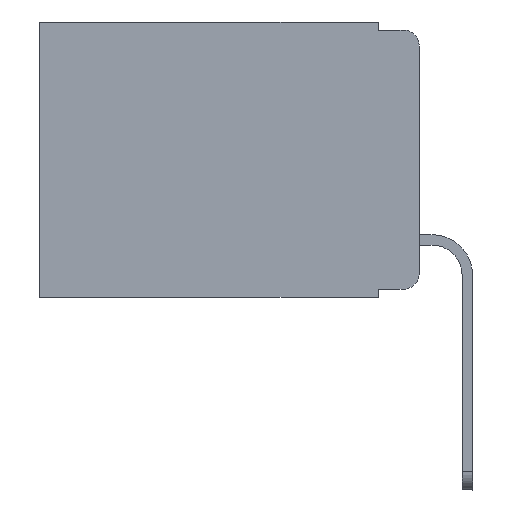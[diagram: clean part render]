
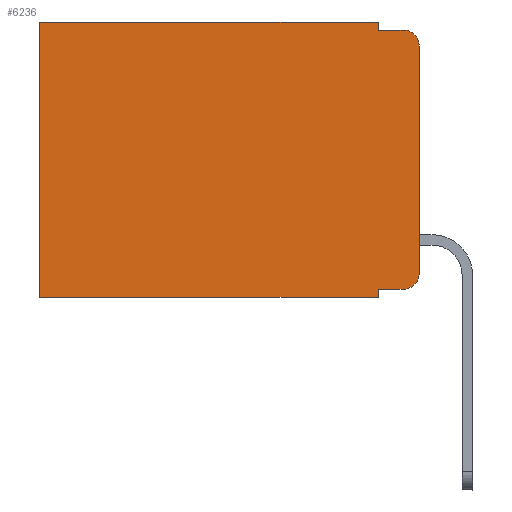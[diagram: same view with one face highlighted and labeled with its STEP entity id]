
A CAD part, left-side view. The second image highlights one B-rep face of the part: STEP entity #6236.
In plain terms, the highlighted planar face has unit normal (-1, 0, 0).
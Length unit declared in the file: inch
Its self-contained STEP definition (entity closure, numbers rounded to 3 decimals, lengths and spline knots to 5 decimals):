
#147 = AXIS2_PLACEMENT_3D ( 'NONE', #1263, #9420, #14792 ) ;
#292 = VECTOR ( 'NONE', #2814, 39.37008 ) ;
#381 = CARTESIAN_POINT ( 'NONE',  ( 0.298, 0., 0. ) ) ;
#407 = CARTESIAN_POINT ( 'NONE',  ( 0.298, 0., -0.03 ) ) ;
#532 = CARTESIAN_POINT ( 'NONE',  ( 0.298, 0.051, -0.333 ) ) ;
#618 = DIRECTION ( 'NONE',  ( 0., 1., 0. ) ) ;
#841 = CARTESIAN_POINT ( 'NONE',  ( 0.298, 0.051, 0. ) ) ;
#1177 = FACE_OUTER_BOUND ( 'NONE', #15107, .T. ) ;
#1263 = CARTESIAN_POINT ( 'NONE',  ( 0.298, 0., 0. ) ) ;
#1312 = DIRECTION ( 'NONE',  ( 0., 0., -1. ) ) ;
#1397 = CARTESIAN_POINT ( 'NONE',  ( 0.298, 0.051, -0.333 ) ) ;
#1492 = CARTESIAN_POINT ( 'NONE',  ( 0.298, 0.051, 0. ) ) ;
#1505 = ORIENTED_EDGE ( 'NONE', *, *, #8779, .F. ) ;
#1575 = VECTOR ( 'NONE', #2455, 39.37008 ) ;
#1596 = CARTESIAN_POINT ( 'NONE',  ( 0.298, 0.02, -0.03 ) ) ;
#1624 = VECTOR ( 'NONE', #5304, 39.37008 ) ;
#1857 = DIRECTION ( 'NONE',  ( 0., -1., 0. ) ) ;
#2455 = DIRECTION ( 'NONE',  ( 0., 0., -1. ) ) ;
#2542 = LINE ( 'NONE', #15718, #1575 ) ;
#2643 = EDGE_CURVE ( 'NONE', #16967, #6027, #7352, .T. ) ;
#2814 = DIRECTION ( 'NONE',  ( 0., 0., -1. ) ) ;
#3098 = ORIENTED_EDGE ( 'NONE', *, *, #8596, .T. ) ;
#3235 = ORIENTED_EDGE ( 'NONE', *, *, #4909, .T. ) ;
#3703 = LINE ( 'NONE', #9099, #292 ) ;
#3715 = EDGE_CURVE ( 'NONE', #4102, #5223, #4600, .T. ) ;
#3789 = CARTESIAN_POINT ( 'NONE',  ( 0.298, 0.02, -0.333 ) ) ;
#3904 = CARTESIAN_POINT ( 'NONE',  ( 0.298, 0., -0.313 ) ) ;
#3988 = EDGE_CURVE ( 'NONE', #6385, #6027, #17222, .T. ) ;
#4102 = VERTEX_POINT ( 'NONE', #1397 ) ;
#4171 = CIRCLE ( 'NONE', #8983, 0.02 ) ;
#4177 = CIRCLE ( 'NONE', #4748, 0.02 ) ;
#4514 = ORIENTED_EDGE ( 'NONE', *, *, #14422, .F. ) ;
#4600 = LINE ( 'NONE', #532, #14358 ) ;
#4748 = AXIS2_PLACEMENT_3D ( 'NONE', #1596, #9482, #13632 ) ;
#4909 = EDGE_CURVE ( 'NONE', #12783, #16648, #4177, .T. ) ;
#4951 = DIRECTION ( 'NONE',  ( -1., 0., 0. ) ) ;
#5069 = CARTESIAN_POINT ( 'NONE',  ( 0.298, 0.473, -0.343 ) ) ;
#5223 = VERTEX_POINT ( 'NONE', #3789 ) ;
#5304 = DIRECTION ( 'NONE',  ( 0., 0., -1. ) ) ;
#5778 = DIRECTION ( 'NONE',  ( 0., 1., 0. ) ) ;
#5978 = CARTESIAN_POINT ( 'NONE',  ( 0.298, 0.02, -0.01 ) ) ;
#5996 = VECTOR ( 'NONE', #16399, 39.37008 ) ;
#6027 = VERTEX_POINT ( 'NONE', #5069 ) ;
#6236 = ADVANCED_FACE ( 'NONE', ( #1177 ), #8004, .F. ) ;
#6385 = VERTEX_POINT ( 'NONE', #11082 ) ;
#6781 = CARTESIAN_POINT ( 'NONE',  ( 0.298, 0.051, -0.01 ) ) ;
#6901 = EDGE_CURVE ( 'NONE', #11610, #9193, #2542, .T. ) ;
#7352 = LINE ( 'NONE', #12740, #13779 ) ;
#8004 = PLANE ( 'NONE',  #147 ) ;
#8048 = ORIENTED_EDGE ( 'NONE', *, *, #3988, .T. ) ;
#8596 = EDGE_CURVE ( 'NONE', #5223, #15212, #4171, .T. ) ;
#8700 = VECTOR ( 'NONE', #5778, 39.37008 ) ;
#8779 = EDGE_CURVE ( 'NONE', #4102, #16967, #10959, .T. ) ;
#8983 = AXIS2_PLACEMENT_3D ( 'NONE', #13003, #4951, #10353 ) ;
#9099 = CARTESIAN_POINT ( 'NONE',  ( 0.298, 0., 0. ) ) ;
#9193 = VERTEX_POINT ( 'NONE', #16239 ) ;
#9297 = ORIENTED_EDGE ( 'NONE', *, *, #3715, .T. ) ;
#9329 = ORIENTED_EDGE ( 'NONE', *, *, #2643, .F. ) ;
#9420 = DIRECTION ( 'NONE',  ( 1., 0., 0. ) ) ;
#9482 = DIRECTION ( 'NONE',  ( -1., 0., 0. ) ) ;
#10351 = ORIENTED_EDGE ( 'NONE', *, *, #12568, .F. ) ;
#10353 = DIRECTION ( 'NONE',  ( 0., 0., -1. ) ) ;
#10511 = CARTESIAN_POINT ( 'NONE',  ( 0.298, 0.473, 0. ) ) ;
#10747 = CARTESIAN_POINT ( 'NONE',  ( 0.298, 0.051, -0.343 ) ) ;
#10959 = LINE ( 'NONE', #1492, #1624 ) ;
#11082 = CARTESIAN_POINT ( 'NONE',  ( 0.298, 0.473, 0. ) ) ;
#11610 = VERTEX_POINT ( 'NONE', #841 ) ;
#12354 = LINE ( 'NONE', #6781, #5996 ) ;
#12568 = EDGE_CURVE ( 'NONE', #12783, #15212, #3703, .T. ) ;
#12643 = ORIENTED_EDGE ( 'NONE', *, *, #17100, .T. ) ;
#12740 = CARTESIAN_POINT ( 'NONE',  ( 0.298, 0., -0.343 ) ) ;
#12783 = VERTEX_POINT ( 'NONE', #407 ) ;
#13003 = CARTESIAN_POINT ( 'NONE',  ( 0.298, 0.02, -0.313 ) ) ;
#13632 = DIRECTION ( 'NONE',  ( 0., 0., -1. ) ) ;
#13659 = LINE ( 'NONE', #381, #8700 ) ;
#13779 = VECTOR ( 'NONE', #618, 39.37008 ) ;
#13963 = ORIENTED_EDGE ( 'NONE', *, *, #6901, .F. ) ;
#14358 = VECTOR ( 'NONE', #1857, 39.37008 ) ;
#14422 = EDGE_CURVE ( 'NONE', #9193, #16648, #12354, .T. ) ;
#14792 = DIRECTION ( 'NONE',  ( 0., 0., -1. ) ) ;
#15107 = EDGE_LOOP ( 'NONE', ( #10351, #3235, #4514, #13963, #12643, #8048, #9329, #1505, #9297, #3098 ) ) ;
#15212 = VERTEX_POINT ( 'NONE', #3904 ) ;
#15718 = CARTESIAN_POINT ( 'NONE',  ( 0.298, 0.051, 0. ) ) ;
#16239 = CARTESIAN_POINT ( 'NONE',  ( 0.298, 0.051, -0.01 ) ) ;
#16399 = DIRECTION ( 'NONE',  ( 0., -1., 0. ) ) ;
#16648 = VERTEX_POINT ( 'NONE', #5978 ) ;
#16967 = VERTEX_POINT ( 'NONE', #10747 ) ;
#17100 = EDGE_CURVE ( 'NONE', #11610, #6385, #13659, .T. ) ;
#17222 = LINE ( 'NONE', #10511, #17240 ) ;
#17240 = VECTOR ( 'NONE', #1312, 39.37008 ) ;
